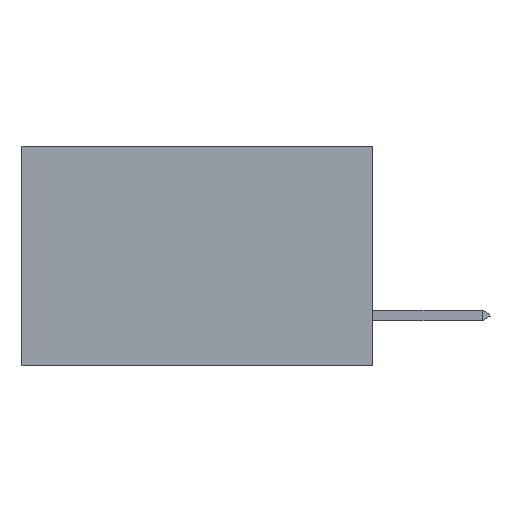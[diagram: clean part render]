
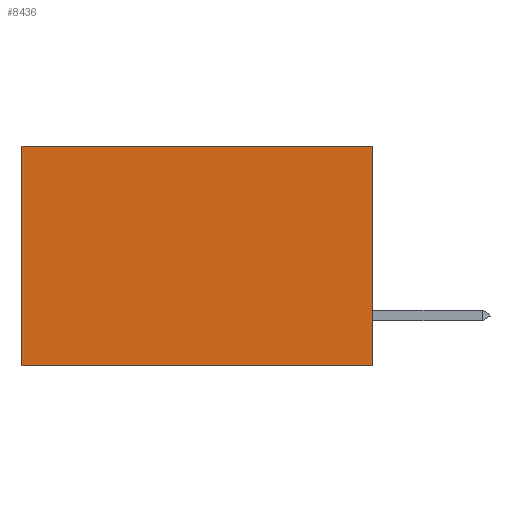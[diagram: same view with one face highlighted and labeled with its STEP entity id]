
A CAD part, left-side view. The second image highlights one B-rep face of the part: STEP entity #8436.
In plain terms, the highlighted planar face has unit normal (-1, 0, 0).
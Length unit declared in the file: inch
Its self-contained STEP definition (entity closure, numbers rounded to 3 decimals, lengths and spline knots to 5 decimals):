
#62 = CARTESIAN_POINT ( 'NONE',  ( 0.277, 0., 0. ) ) ;
#491 = VERTEX_POINT ( 'NONE', #5393 ) ;
#1276 = VECTOR ( 'NONE', #11031, 39.37008 ) ;
#1323 = ORIENTED_EDGE ( 'NONE', *, *, #13993, .F. ) ;
#1802 = EDGE_CURVE ( 'NONE', #4330, #491, #14977, .T. ) ;
#1972 = PLANE ( 'NONE',  #8011 ) ;
#2878 = VERTEX_POINT ( 'NONE', #7705 ) ;
#3034 = VECTOR ( 'NONE', #4922, 39.37008 ) ;
#3413 = LINE ( 'NONE', #8553, #3034 ) ;
#3647 = VERTEX_POINT ( 'NONE', #10390 ) ;
#3729 = VECTOR ( 'NONE', #14720, 39.37008 ) ;
#4330 = VERTEX_POINT ( 'NONE', #15183 ) ;
#4424 = DIRECTION ( 'NONE',  ( 1., 0., 0. ) ) ;
#4532 = LINE ( 'NONE', #62, #1276 ) ;
#4739 = ORIENTED_EDGE ( 'NONE', *, *, #1802, .T. ) ;
#4922 = DIRECTION ( 'NONE',  ( 0., 1., 0. ) ) ;
#5326 = ORIENTED_EDGE ( 'NONE', *, *, #10981, .F. ) ;
#5393 = CARTESIAN_POINT ( 'NONE',  ( 0.277, 0.59, -0.37 ) ) ;
#6217 = CARTESIAN_POINT ( 'NONE',  ( 0.277, 0., -0.37 ) ) ;
#6697 = FACE_OUTER_BOUND ( 'NONE', #11797, .T. ) ;
#7705 = CARTESIAN_POINT ( 'NONE',  ( 0.277, 0., -0.37 ) ) ;
#8011 = AXIS2_PLACEMENT_3D ( 'NONE', #11650, #4424, #12918 ) ;
#8256 = ORIENTED_EDGE ( 'NONE', *, *, #10067, .T. ) ;
#8436 = ADVANCED_FACE ( 'NONE', ( #6697 ), #1972, .F. ) ;
#8553 = CARTESIAN_POINT ( 'NONE',  ( 0.277, 0., -0.37 ) ) ;
#10067 = EDGE_CURVE ( 'NONE', #3647, #4330, #4532, .T. ) ;
#10390 = CARTESIAN_POINT ( 'NONE',  ( 0.277, 0., 0. ) ) ;
#10981 = EDGE_CURVE ( 'NONE', #3647, #2878, #13056, .T. ) ;
#11031 = DIRECTION ( 'NONE',  ( 0., 1., 0. ) ) ;
#11650 = CARTESIAN_POINT ( 'NONE',  ( 0.277, 0., -0.37 ) ) ;
#11797 = EDGE_LOOP ( 'NONE', ( #4739, #1323, #5326, #8256 ) ) ;
#12918 = DIRECTION ( 'NONE',  ( 0., 0., -1. ) ) ;
#13056 = LINE ( 'NONE', #6217, #3729 ) ;
#13993 = EDGE_CURVE ( 'NONE', #2878, #491, #3413, .T. ) ;
#14516 = CARTESIAN_POINT ( 'NONE',  ( 0.277, 0.59, -0.37 ) ) ;
#14589 = VECTOR ( 'NONE', #14635, 39.37008 ) ;
#14635 = DIRECTION ( 'NONE',  ( 0., 0., -1. ) ) ;
#14720 = DIRECTION ( 'NONE',  ( 0., 0., -1. ) ) ;
#14977 = LINE ( 'NONE', #14516, #14589 ) ;
#15183 = CARTESIAN_POINT ( 'NONE',  ( 0.277, 0.59, 0. ) ) ;
